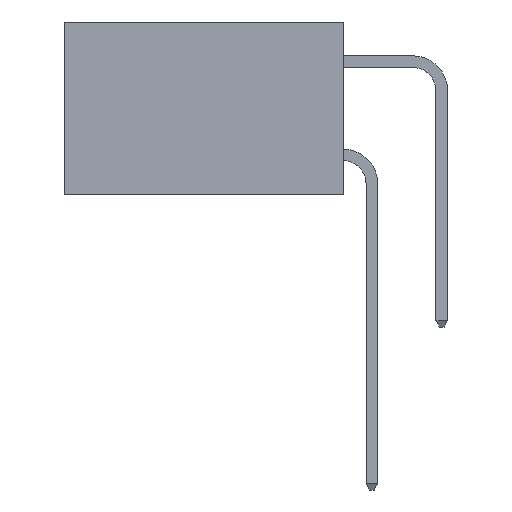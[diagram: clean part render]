
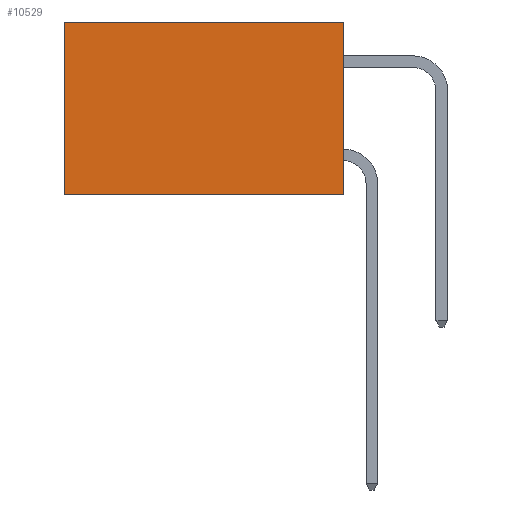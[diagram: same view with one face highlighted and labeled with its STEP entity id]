
A CAD part, left-side view. The second image highlights one B-rep face of the part: STEP entity #10529.
In plain terms, the highlighted planar face has unit normal (-1, 0, 0).
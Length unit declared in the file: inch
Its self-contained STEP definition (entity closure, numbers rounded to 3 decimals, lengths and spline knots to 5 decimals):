
#38 = VERTEX_POINT ( 'NONE', #10197 ) ;
#281 = PLANE ( 'NONE',  #19246 ) ;
#2005 = DIRECTION ( 'NONE',  ( 0., 0., -1. ) ) ;
#2187 = EDGE_CURVE ( 'NONE', #8922, #8437, #7698, .T. ) ;
#2216 = LINE ( 'NONE', #18177, #13921 ) ;
#2280 = EDGE_CURVE ( 'NONE', #10587, #8922, #2216, .T. ) ;
#2310 = EDGE_CURVE ( 'NONE', #38, #8437, #13393, .T. ) ;
#2945 = CARTESIAN_POINT ( 'NONE',  ( 0.2615, 0.6, -0.37 ) ) ;
#5270 = CARTESIAN_POINT ( 'NONE',  ( 0.2615, 0., -0.37 ) ) ;
#5646 = ORIENTED_EDGE ( 'NONE', *, *, #2280, .F. ) ;
#5795 = ORIENTED_EDGE ( 'NONE', *, *, #2187, .F. ) ;
#7119 = CARTESIAN_POINT ( 'NONE',  ( 0.2615, 0., 0. ) ) ;
#7181 = VECTOR ( 'NONE', #11639, 39.37008 ) ;
#7292 = DIRECTION ( 'NONE',  ( 0., 0., -1. ) ) ;
#7698 = LINE ( 'NONE', #19425, #7181 ) ;
#8161 = CARTESIAN_POINT ( 'NONE',  ( 0.2615, 0.6, -0.37 ) ) ;
#8437 = VERTEX_POINT ( 'NONE', #2945 ) ;
#8891 = DIRECTION ( 'NONE',  ( 0., 0., -1. ) ) ;
#8922 = VERTEX_POINT ( 'NONE', #10872 ) ;
#9805 = ORIENTED_EDGE ( 'NONE', *, *, #2310, .T. ) ;
#10197 = CARTESIAN_POINT ( 'NONE',  ( 0.2615, 0.6, 0. ) ) ;
#10529 = ADVANCED_FACE ( 'NONE', ( #13317 ), #281, .F. ) ;
#10587 = VERTEX_POINT ( 'NONE', #7119 ) ;
#10872 = CARTESIAN_POINT ( 'NONE',  ( 0.2615, 0., -0.37 ) ) ;
#11639 = DIRECTION ( 'NONE',  ( 0., 1., 0. ) ) ;
#11981 = DIRECTION ( 'NONE',  ( 1., 0., 0. ) ) ;
#11990 = ORIENTED_EDGE ( 'NONE', *, *, #14834, .T. ) ;
#12877 = DIRECTION ( 'NONE',  ( 0., 1., 0. ) ) ;
#13317 = FACE_OUTER_BOUND ( 'NONE', #18206, .T. ) ;
#13393 = LINE ( 'NONE', #8161, #18727 ) ;
#13921 = VECTOR ( 'NONE', #8891, 39.37008 ) ;
#14478 = CARTESIAN_POINT ( 'NONE',  ( 0.2615, 0., 0. ) ) ;
#14834 = EDGE_CURVE ( 'NONE', #10587, #38, #20340, .T. ) ;
#16058 = VECTOR ( 'NONE', #12877, 39.37008 ) ;
#18177 = CARTESIAN_POINT ( 'NONE',  ( 0.2615, 0., -0.37 ) ) ;
#18206 = EDGE_LOOP ( 'NONE', ( #9805, #5795, #5646, #11990 ) ) ;
#18727 = VECTOR ( 'NONE', #7292, 39.37008 ) ;
#19246 = AXIS2_PLACEMENT_3D ( 'NONE', #5270, #11981, #2005 ) ;
#19425 = CARTESIAN_POINT ( 'NONE',  ( 0.2615, 0., -0.37 ) ) ;
#20340 = LINE ( 'NONE', #14478, #16058 ) ;
